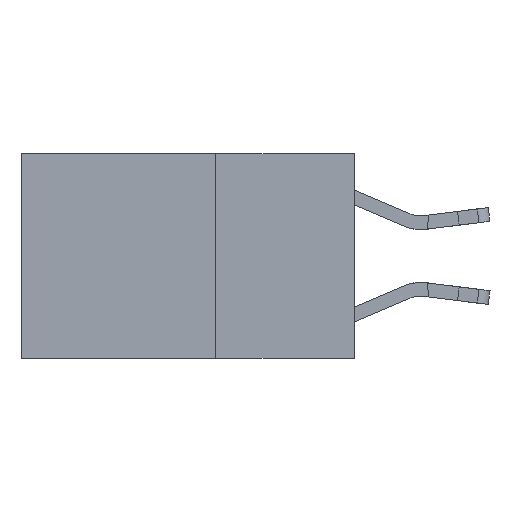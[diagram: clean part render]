
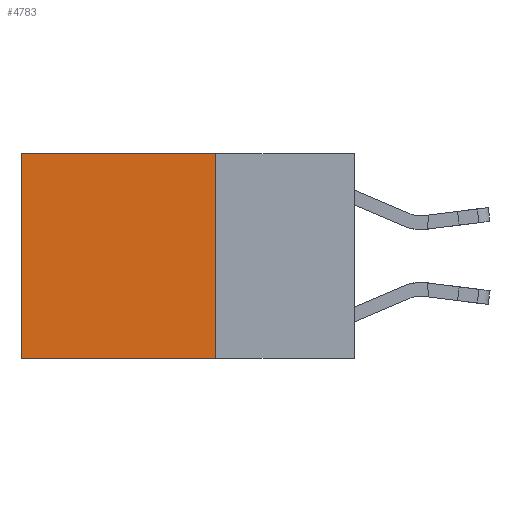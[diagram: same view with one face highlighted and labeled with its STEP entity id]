
A CAD part, left-side view. The second image highlights one B-rep face of the part: STEP entity #4783.
In plain terms, the highlighted planar face has unit normal (-1, 0, 0).
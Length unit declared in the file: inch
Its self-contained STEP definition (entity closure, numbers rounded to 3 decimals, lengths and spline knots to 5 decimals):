
#18 = CARTESIAN_POINT ( 'NONE',  ( 0.2625, 0.25, 0. ) ) ;
#145 = LINE ( 'NONE', #519, #3170 ) ;
#519 = CARTESIAN_POINT ( 'NONE',  ( 0.2625, 0.25, 0. ) ) ;
#1208 = AXIS2_PLACEMENT_3D ( 'NONE', #18, #8929, #1366 ) ;
#1366 = DIRECTION ( 'NONE',  ( 0., 0., -1. ) ) ;
#1673 = ORIENTED_EDGE ( 'NONE', *, *, #1990, .T. ) ;
#1730 = CARTESIAN_POINT ( 'NONE',  ( 0.2625, 0.6, -0.37 ) ) ;
#1990 = EDGE_CURVE ( 'NONE', #15241, #3370, #6448, .T. ) ;
#3135 = ORIENTED_EDGE ( 'NONE', *, *, #11116, .F. ) ;
#3170 = VECTOR ( 'NONE', #5598, 39.37008 ) ;
#3370 = VERTEX_POINT ( 'NONE', #1730 ) ;
#3956 = DIRECTION ( 'NONE',  ( 0., 0., -1. ) ) ;
#4101 = EDGE_CURVE ( 'NONE', #11940, #3370, #9083, .T. ) ;
#4396 = ORIENTED_EDGE ( 'NONE', *, *, #9715, .T. ) ;
#4783 = ADVANCED_FACE ( 'NONE', ( #9266 ), #7669, .F. ) ;
#4931 = LINE ( 'NONE', #5105, #7859 ) ;
#5105 = CARTESIAN_POINT ( 'NONE',  ( 0.2625, 0.25, 0. ) ) ;
#5598 = DIRECTION ( 'NONE',  ( 0., 1., 0. ) ) ;
#5906 = CARTESIAN_POINT ( 'NONE',  ( 0.2625, 0.25, -0.37 ) ) ;
#6448 = LINE ( 'NONE', #6497, #16061 ) ;
#6497 = CARTESIAN_POINT ( 'NONE',  ( 0.2625, 0.6, 0. ) ) ;
#7419 = CARTESIAN_POINT ( 'NONE',  ( 0.2625, 0.25, -0.37 ) ) ;
#7669 = PLANE ( 'NONE',  #1208 ) ;
#7859 = VECTOR ( 'NONE', #13907, 39.37008 ) ;
#8232 = ORIENTED_EDGE ( 'NONE', *, *, #4101, .F. ) ;
#8825 = CARTESIAN_POINT ( 'NONE',  ( 0.2625, 0.6, 0. ) ) ;
#8929 = DIRECTION ( 'NONE',  ( 1., 0., 0. ) ) ;
#9083 = LINE ( 'NONE', #7419, #12117 ) ;
#9242 = EDGE_LOOP ( 'NONE', ( #1673, #8232, #3135, #4396 ) ) ;
#9266 = FACE_OUTER_BOUND ( 'NONE', #9242, .T. ) ;
#9715 = EDGE_CURVE ( 'NONE', #13848, #15241, #145, .T. ) ;
#9902 = DIRECTION ( 'NONE',  ( 0., 1., 0. ) ) ;
#11116 = EDGE_CURVE ( 'NONE', #13848, #11940, #4931, .T. ) ;
#11940 = VERTEX_POINT ( 'NONE', #5906 ) ;
#12117 = VECTOR ( 'NONE', #9902, 39.37008 ) ;
#13848 = VERTEX_POINT ( 'NONE', #16257 ) ;
#13907 = DIRECTION ( 'NONE',  ( 0., 0., -1. ) ) ;
#15241 = VERTEX_POINT ( 'NONE', #8825 ) ;
#16061 = VECTOR ( 'NONE', #3956, 39.37008 ) ;
#16257 = CARTESIAN_POINT ( 'NONE',  ( 0.2625, 0.25, 0. ) ) ;
